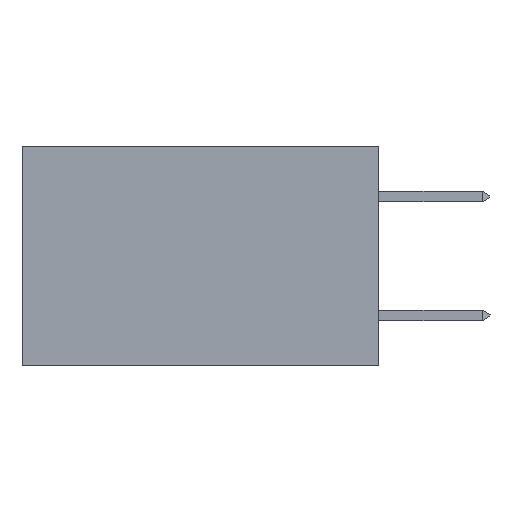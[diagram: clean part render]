
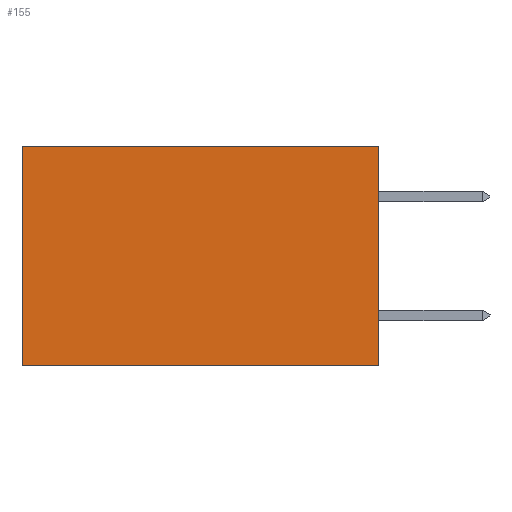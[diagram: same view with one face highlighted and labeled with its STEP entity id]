
A CAD part, left-side view. The second image highlights one B-rep face of the part: STEP entity #155.
In plain terms, the highlighted planar face has unit normal (-1, 0, 0).
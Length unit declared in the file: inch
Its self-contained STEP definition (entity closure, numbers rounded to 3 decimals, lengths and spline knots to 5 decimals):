
#155 = ADVANCED_FACE ( 'NONE', ( #20202 ), #4343, .F. ) ;
#199 = DIRECTION ( 'NONE',  ( 0., 0., -1. ) ) ;
#1304 = CARTESIAN_POINT ( 'NONE',  ( 0.298, 0., 0. ) ) ;
#1333 = CARTESIAN_POINT ( 'NONE',  ( 0.298, 0., -0.37 ) ) ;
#2732 = CARTESIAN_POINT ( 'NONE',  ( 0.298, 0., 0. ) ) ;
#3036 = DIRECTION ( 'NONE',  ( 0., 1., 0. ) ) ;
#4343 = PLANE ( 'NONE',  #11850 ) ;
#5572 = VERTEX_POINT ( 'NONE', #14667 ) ;
#6034 = ORIENTED_EDGE ( 'NONE', *, *, #8813, .F. ) ;
#7702 = VECTOR ( 'NONE', #199, 39.37008 ) ;
#7967 = LINE ( 'NONE', #17889, #7702 ) ;
#8253 = LINE ( 'NONE', #1304, #16002 ) ;
#8813 = EDGE_CURVE ( 'NONE', #10862, #19942, #7967, .T. ) ;
#9204 = LINE ( 'NONE', #1333, #20483 ) ;
#9551 = EDGE_CURVE ( 'NONE', #5572, #12638, #17268, .T. ) ;
#10411 = ORIENTED_EDGE ( 'NONE', *, *, #9551, .T. ) ;
#10862 = VERTEX_POINT ( 'NONE', #15606 ) ;
#11502 = DIRECTION ( 'NONE',  ( 0., 0., -1. ) ) ;
#11608 = EDGE_CURVE ( 'NONE', #19942, #12638, #9204, .T. ) ;
#11850 = AXIS2_PLACEMENT_3D ( 'NONE', #2732, #13966, #20448 ) ;
#12638 = VERTEX_POINT ( 'NONE', #15463 ) ;
#13966 = DIRECTION ( 'NONE',  ( 1., 0., 0. ) ) ;
#14213 = DIRECTION ( 'NONE',  ( 0., 1., 0. ) ) ;
#14631 = CARTESIAN_POINT ( 'NONE',  ( 0.298, 0.6, 0. ) ) ;
#14667 = CARTESIAN_POINT ( 'NONE',  ( 0.298, 0.6, 0. ) ) ;
#15411 = EDGE_CURVE ( 'NONE', #10862, #5572, #8253, .T. ) ;
#15463 = CARTESIAN_POINT ( 'NONE',  ( 0.298, 0.6, -0.37 ) ) ;
#15606 = CARTESIAN_POINT ( 'NONE',  ( 0.298, 0., 0. ) ) ;
#16002 = VECTOR ( 'NONE', #3036, 39.37008 ) ;
#16619 = CARTESIAN_POINT ( 'NONE',  ( 0.298, 0., -0.37 ) ) ;
#17268 = LINE ( 'NONE', #14631, #20031 ) ;
#17888 = EDGE_LOOP ( 'NONE', ( #10411, #18398, #6034, #20573 ) ) ;
#17889 = CARTESIAN_POINT ( 'NONE',  ( 0.298, 0., 0. ) ) ;
#18398 = ORIENTED_EDGE ( 'NONE', *, *, #11608, .F. ) ;
#19942 = VERTEX_POINT ( 'NONE', #16619 ) ;
#20031 = VECTOR ( 'NONE', #11502, 39.37008 ) ;
#20202 = FACE_OUTER_BOUND ( 'NONE', #17888, .T. ) ;
#20448 = DIRECTION ( 'NONE',  ( 0., 0., -1. ) ) ;
#20483 = VECTOR ( 'NONE', #14213, 39.37008 ) ;
#20573 = ORIENTED_EDGE ( 'NONE', *, *, #15411, .T. ) ;
